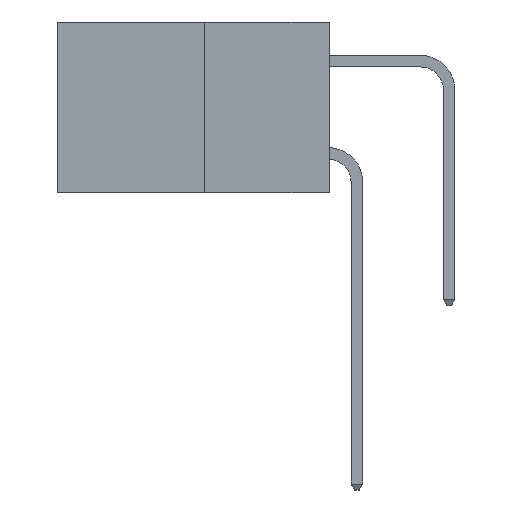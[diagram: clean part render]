
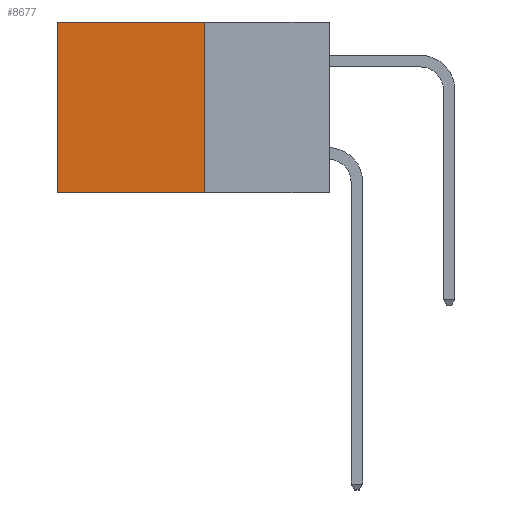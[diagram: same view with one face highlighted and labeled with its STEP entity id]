
A CAD part, left-side view. The second image highlights one B-rep face of the part: STEP entity #8677.
In plain terms, the highlighted planar face has unit normal (-1, 0, 0).
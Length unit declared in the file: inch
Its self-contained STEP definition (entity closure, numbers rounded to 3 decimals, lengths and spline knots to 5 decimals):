
#872 = VERTEX_POINT ( 'NONE', #5661 ) ;
#979 = ORIENTED_EDGE ( 'NONE', *, *, #1246, .F. ) ;
#1097 = ORIENTED_EDGE ( 'NONE', *, *, #11757, .T. ) ;
#1246 = EDGE_CURVE ( 'NONE', #4696, #872, #8135, .T. ) ;
#1629 = DIRECTION ( 'NONE',  ( 0., 0., -1. ) ) ;
#2068 = EDGE_CURVE ( 'NONE', #14160, #872, #12951, .T. ) ;
#2643 = LINE ( 'NONE', #12871, #8197 ) ;
#3446 = CARTESIAN_POINT ( 'NONE',  ( 0.277, 0.27, 0. ) ) ;
#3651 = CARTESIAN_POINT ( 'NONE',  ( 0.277, 0.27, -0.37 ) ) ;
#3957 = FACE_OUTER_BOUND ( 'NONE', #12599, .T. ) ;
#4005 = VECTOR ( 'NONE', #1629, 39.37008 ) ;
#4260 = CARTESIAN_POINT ( 'NONE',  ( 0.277, 0.27, -0.37 ) ) ;
#4561 = DIRECTION ( 'NONE',  ( 0., 1., 0. ) ) ;
#4696 = VERTEX_POINT ( 'NONE', #10664 ) ;
#4740 = DIRECTION ( 'NONE',  ( 0., 0., -1. ) ) ;
#4782 = CARTESIAN_POINT ( 'NONE',  ( 0.277, 0.27, 0. ) ) ;
#5453 = AXIS2_PLACEMENT_3D ( 'NONE', #3651, #11478, #4740 ) ;
#5661 = CARTESIAN_POINT ( 'NONE',  ( 0.277, 0.59, -0.37 ) ) ;
#7264 = DIRECTION ( 'NONE',  ( 0., 1., 0. ) ) ;
#7416 = VERTEX_POINT ( 'NONE', #4782 ) ;
#8135 = LINE ( 'NONE', #4260, #10791 ) ;
#8188 = EDGE_CURVE ( 'NONE', #7416, #4696, #2643, .T. ) ;
#8197 = VECTOR ( 'NONE', #8371, 39.37008 ) ;
#8215 = VECTOR ( 'NONE', #4561, 39.37008 ) ;
#8332 = CARTESIAN_POINT ( 'NONE',  ( 0.277, 0.59, 0. ) ) ;
#8371 = DIRECTION ( 'NONE',  ( 0., 0., -1. ) ) ;
#8677 = ADVANCED_FACE ( 'NONE', ( #3957 ), #10377, .F. ) ;
#9837 = ORIENTED_EDGE ( 'NONE', *, *, #2068, .T. ) ;
#10377 = PLANE ( 'NONE',  #5453 ) ;
#10481 = ORIENTED_EDGE ( 'NONE', *, *, #8188, .F. ) ;
#10664 = CARTESIAN_POINT ( 'NONE',  ( 0.277, 0.27, -0.37 ) ) ;
#10791 = VECTOR ( 'NONE', #7264, 39.37008 ) ;
#11478 = DIRECTION ( 'NONE',  ( 1., 0., 0. ) ) ;
#11757 = EDGE_CURVE ( 'NONE', #7416, #14160, #13821, .T. ) ;
#12599 = EDGE_LOOP ( 'NONE', ( #9837, #979, #10481, #1097 ) ) ;
#12871 = CARTESIAN_POINT ( 'NONE',  ( 0.277, 0.27, -0.37 ) ) ;
#12951 = LINE ( 'NONE', #14430, #4005 ) ;
#13821 = LINE ( 'NONE', #3446, #8215 ) ;
#14160 = VERTEX_POINT ( 'NONE', #8332 ) ;
#14430 = CARTESIAN_POINT ( 'NONE',  ( 0.277, 0.59, -0.37 ) ) ;
